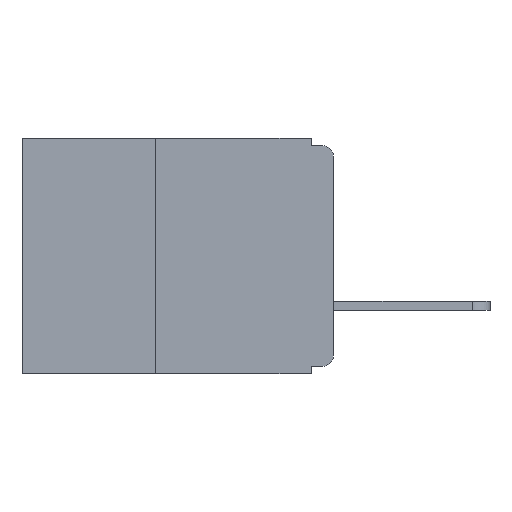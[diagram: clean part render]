
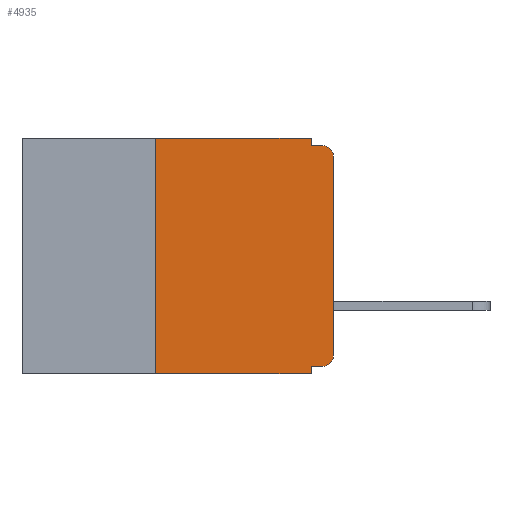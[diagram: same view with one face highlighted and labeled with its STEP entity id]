
A CAD part, left-side view. The second image highlights one B-rep face of the part: STEP entity #4935.
In plain terms, the highlighted planar face has unit normal (-1, 0, 0).
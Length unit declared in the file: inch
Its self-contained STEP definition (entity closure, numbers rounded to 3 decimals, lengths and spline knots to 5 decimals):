
#132 = VERTEX_POINT ( 'NONE', #28568 ) ;
#164 = VECTOR ( 'NONE', #7724, 39.37008 ) ;
#761 = CARTESIAN_POINT ( 'NONE',  ( 0., 0., 0. ) ) ;
#967 = DIRECTION ( 'NONE',  ( 0., 1., 0. ) ) ;
#1356 = VECTOR ( 'NONE', #7474, 39.37008 ) ;
#1475 = DIRECTION ( 'NONE',  ( 0., -1., 0. ) ) ;
#1975 = DIRECTION ( 'NONE',  ( 0., -1., 0. ) ) ;
#2001 = VERTEX_POINT ( 'NONE', #10617 ) ;
#2016 = CARTESIAN_POINT ( 'NONE',  ( 0., 0.015, -0.305 ) ) ;
#2459 = DIRECTION ( 'NONE',  ( 0., 0., -1. ) ) ;
#3542 = CIRCLE ( 'NONE', #17548, 0.015 ) ;
#3624 = ORIENTED_EDGE ( 'NONE', *, *, #23581, .F. ) ;
#3995 = ORIENTED_EDGE ( 'NONE', *, *, #6614, .T. ) ;
#4003 = CARTESIAN_POINT ( 'NONE',  ( 0., 0.015, -0.025 ) ) ;
#4082 = EDGE_LOOP ( 'NONE', ( #5365, #27155, #24083, #17166, #19794, #8448, #3995, #3624, #25489, #4144 ) ) ;
#4144 = ORIENTED_EDGE ( 'NONE', *, *, #25982, .T. ) ;
#4357 = DIRECTION ( 'NONE',  ( 0., 0., -1. ) ) ;
#4935 = ADVANCED_FACE ( 'NONE', ( #7359 ), #25260, .F. ) ;
#5365 = ORIENTED_EDGE ( 'NONE', *, *, #16690, .T. ) ;
#6325 = DIRECTION ( 'NONE',  ( 0., 0., -1. ) ) ;
#6614 = EDGE_CURVE ( 'NONE', #15314, #28812, #25604, .T. ) ;
#7013 = VECTOR ( 'NONE', #10911, 39.37008 ) ;
#7208 = CARTESIAN_POINT ( 'NONE',  ( 0., 0.25, -0.33 ) ) ;
#7212 = CARTESIAN_POINT ( 'NONE',  ( 0., 0.031, 0. ) ) ;
#7359 = FACE_OUTER_BOUND ( 'NONE', #4082, .T. ) ;
#7474 = DIRECTION ( 'NONE',  ( 0., 0., 1. ) ) ;
#7724 = DIRECTION ( 'NONE',  ( 0., 0., 1. ) ) ;
#8163 = LINE ( 'NONE', #13016, #13606 ) ;
#8448 = ORIENTED_EDGE ( 'NONE', *, *, #12416, .F. ) ;
#8513 = CARTESIAN_POINT ( 'NONE',  ( 0., 0.031, -0.32 ) ) ;
#8525 = VECTOR ( 'NONE', #967, 39.37008 ) ;
#9001 = CARTESIAN_POINT ( 'NONE',  ( 0., 0.437, -0.33 ) ) ;
#10617 = CARTESIAN_POINT ( 'NONE',  ( 0., 0.015, -0.32 ) ) ;
#10911 = DIRECTION ( 'NONE',  ( 0., 0., -1. ) ) ;
#11518 = DIRECTION ( 'NONE',  ( 1., 0., 0. ) ) ;
#12122 = VERTEX_POINT ( 'NONE', #8513 ) ;
#12416 = EDGE_CURVE ( 'NONE', #15314, #23153, #25861, .T. ) ;
#12503 = CARTESIAN_POINT ( 'NONE',  ( 0., 0., -0.32 ) ) ;
#13016 = CARTESIAN_POINT ( 'NONE',  ( 0., 0., -0.01 ) ) ;
#13232 = LINE ( 'NONE', #761, #164 ) ;
#13282 = CARTESIAN_POINT ( 'NONE',  ( 0., 0., -0.025 ) ) ;
#13308 = EDGE_CURVE ( 'NONE', #28597, #132, #8163, .T. ) ;
#13516 = LINE ( 'NONE', #27214, #18178 ) ;
#13606 = VECTOR ( 'NONE', #1475, 39.37008 ) ;
#13898 = LINE ( 'NONE', #22374, #7013 ) ;
#14005 = VERTEX_POINT ( 'NONE', #13282 ) ;
#15040 = EDGE_CURVE ( 'NONE', #14005, #132, #3542, .T. ) ;
#15106 = CARTESIAN_POINT ( 'NONE',  ( 0., 0.031, 0. ) ) ;
#15314 = VERTEX_POINT ( 'NONE', #7208 ) ;
#16000 = VECTOR ( 'NONE', #2459, 39.37008 ) ;
#16690 = EDGE_CURVE ( 'NONE', #20819, #14005, #13232, .T. ) ;
#16918 = CARTESIAN_POINT ( 'NONE',  ( 0., 0.031, -0.01 ) ) ;
#17166 = ORIENTED_EDGE ( 'NONE', *, *, #24420, .F. ) ;
#17548 = AXIS2_PLACEMENT_3D ( 'NONE', #4003, #20135, #6325 ) ;
#18176 = DIRECTION ( 'NONE',  ( -1., 0., 0. ) ) ;
#18178 = VECTOR ( 'NONE', #1975, 39.37008 ) ;
#19245 = AXIS2_PLACEMENT_3D ( 'NONE', #20671, #11518, #27529 ) ;
#19794 = ORIENTED_EDGE ( 'NONE', *, *, #24273, .F. ) ;
#20076 = LINE ( 'NONE', #12503, #8525 ) ;
#20135 = DIRECTION ( 'NONE',  ( -1., 0., 0. ) ) ;
#20249 = VECTOR ( 'NONE', #27366, 39.37008 ) ;
#20671 = CARTESIAN_POINT ( 'NONE',  ( 0., 0.437, 0. ) ) ;
#20819 = VERTEX_POINT ( 'NONE', #26050 ) ;
#22374 = CARTESIAN_POINT ( 'NONE',  ( 0., 0.031, -0.33 ) ) ;
#22733 = EDGE_CURVE ( 'NONE', #2001, #12122, #20076, .T. ) ;
#22801 = VERTEX_POINT ( 'NONE', #15106 ) ;
#23153 = VERTEX_POINT ( 'NONE', #25511 ) ;
#23581 = EDGE_CURVE ( 'NONE', #12122, #28812, #13898, .T. ) ;
#24083 = ORIENTED_EDGE ( 'NONE', *, *, #13308, .F. ) ;
#24273 = EDGE_CURVE ( 'NONE', #23153, #22801, #13516, .T. ) ;
#24420 = EDGE_CURVE ( 'NONE', #22801, #28597, #26749, .T. ) ;
#24538 = CARTESIAN_POINT ( 'NONE',  ( 0., 0.031, -0.33 ) ) ;
#25260 = PLANE ( 'NONE',  #19245 ) ;
#25268 = CIRCLE ( 'NONE', #28573, 0.015 ) ;
#25489 = ORIENTED_EDGE ( 'NONE', *, *, #22733, .F. ) ;
#25511 = CARTESIAN_POINT ( 'NONE',  ( 0., 0.25, 0. ) ) ;
#25604 = LINE ( 'NONE', #9001, #20249 ) ;
#25861 = LINE ( 'NONE', #25891, #1356 ) ;
#25891 = CARTESIAN_POINT ( 'NONE',  ( 0., 0.25, -0.33 ) ) ;
#25982 = EDGE_CURVE ( 'NONE', #2001, #20819, #25268, .T. ) ;
#26050 = CARTESIAN_POINT ( 'NONE',  ( 0., 0., -0.305 ) ) ;
#26749 = LINE ( 'NONE', #7212, #16000 ) ;
#27155 = ORIENTED_EDGE ( 'NONE', *, *, #15040, .T. ) ;
#27214 = CARTESIAN_POINT ( 'NONE',  ( 0., 0.437, 0. ) ) ;
#27366 = DIRECTION ( 'NONE',  ( 0., -1., 0. ) ) ;
#27529 = DIRECTION ( 'NONE',  ( 0., 0., -1. ) ) ;
#28568 = CARTESIAN_POINT ( 'NONE',  ( 0., 0.015, -0.01 ) ) ;
#28573 = AXIS2_PLACEMENT_3D ( 'NONE', #2016, #18176, #4357 ) ;
#28597 = VERTEX_POINT ( 'NONE', #16918 ) ;
#28812 = VERTEX_POINT ( 'NONE', #24538 ) ;
